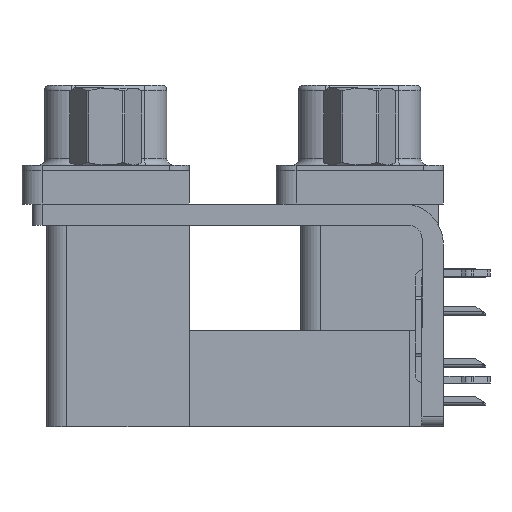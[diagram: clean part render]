
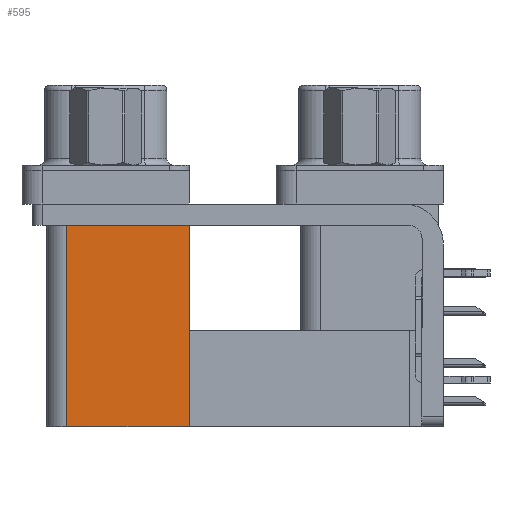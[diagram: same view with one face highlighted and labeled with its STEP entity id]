
A CAD part, left-side view. The second image highlights one B-rep face of the part: STEP entity #595.
In plain terms, the highlighted planar face has unit normal (-1, 0, 0).
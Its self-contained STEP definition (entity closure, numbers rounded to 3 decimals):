
#595 = ADVANCED_FACE ( 'NONE', ( #23436 ), #26953, .F. ) ;
#788 = EDGE_LOOP ( 'NONE', ( #10792, #31267, #27528, #38430 ) ) ;
#1487 = CARTESIAN_POINT ( 'NONE',  ( 3.765, 12.775, -2.5 ) ) ;
#1530 = LINE ( 'NONE', #5298, #18020 ) ;
#4070 = DIRECTION ( 'NONE',  ( 0., 1., 0. ) ) ;
#4829 = DIRECTION ( 'NONE',  ( 0., 0., 1. ) ) ;
#5298 = CARTESIAN_POINT ( 'NONE',  ( 3.765, 12.775, -19.2 ) ) ;
#5978 = CARTESIAN_POINT ( 'NONE',  ( 3.765, 12.775, -19.2 ) ) ;
#6158 = VECTOR ( 'NONE', #4070, 1000. ) ;
#10192 = CARTESIAN_POINT ( 'NONE',  ( 3.765, 21.975, -2.5 ) ) ;
#10792 = ORIENTED_EDGE ( 'NONE', *, *, #21336, .T. ) ;
#13986 = CARTESIAN_POINT ( 'NONE',  ( 3.765, 12.775, -19.2 ) ) ;
#15316 = EDGE_CURVE ( 'NONE', #24178, #31083, #25416, .T. ) ;
#17644 = VECTOR ( 'NONE', #28973, 1000. ) ;
#17930 = DIRECTION ( 'NONE',  ( 1., 0., 0. ) ) ;
#18020 = VECTOR ( 'NONE', #37890, 1000. ) ;
#18529 = EDGE_CURVE ( 'NONE', #24278, #24178, #1530, .T. ) ;
#20688 = DIRECTION ( 'NONE',  ( 0., 0., -1. ) ) ;
#21336 = EDGE_CURVE ( 'NONE', #29347, #31083, #34099, .T. ) ;
#22881 = LINE ( 'NONE', #34858, #17644 ) ;
#23436 = FACE_OUTER_BOUND ( 'NONE', #788, .T. ) ;
#24178 = VERTEX_POINT ( 'NONE', #27534 ) ;
#24278 = VERTEX_POINT ( 'NONE', #13986 ) ;
#25416 = LINE ( 'NONE', #31732, #33526 ) ;
#26953 = PLANE ( 'NONE',  #29411 ) ;
#27528 = ORIENTED_EDGE ( 'NONE', *, *, #18529, .F. ) ;
#27534 = CARTESIAN_POINT ( 'NONE',  ( 3.765, 21.975, -19.2 ) ) ;
#28973 = DIRECTION ( 'NONE',  ( 0., 0., 1. ) ) ;
#29347 = VERTEX_POINT ( 'NONE', #31328 ) ;
#29411 = AXIS2_PLACEMENT_3D ( 'NONE', #5978, #17930, #20688 ) ;
#31083 = VERTEX_POINT ( 'NONE', #10192 ) ;
#31267 = ORIENTED_EDGE ( 'NONE', *, *, #15316, .F. ) ;
#31328 = CARTESIAN_POINT ( 'NONE',  ( 3.765, 12.775, -2.5 ) ) ;
#31732 = CARTESIAN_POINT ( 'NONE',  ( 3.765, 21.975, -19.2 ) ) ;
#33526 = VECTOR ( 'NONE', #4829, 1000. ) ;
#34099 = LINE ( 'NONE', #1487, #6158 ) ;
#34858 = CARTESIAN_POINT ( 'NONE',  ( 3.765, 12.775, -19.2 ) ) ;
#35563 = EDGE_CURVE ( 'NONE', #24278, #29347, #22881, .T. ) ;
#37890 = DIRECTION ( 'NONE',  ( 0., 1., 0. ) ) ;
#38430 = ORIENTED_EDGE ( 'NONE', *, *, #35563, .T. ) ;
